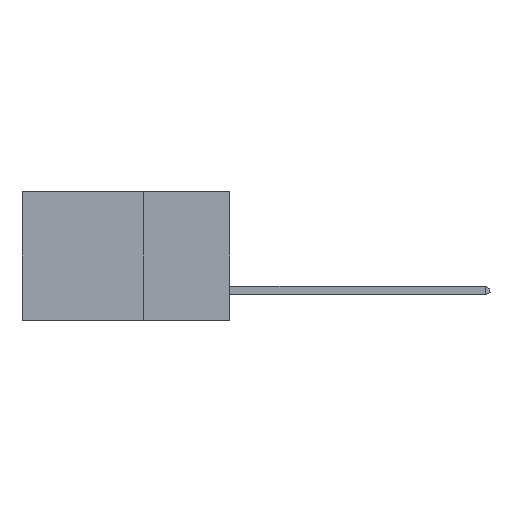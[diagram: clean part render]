
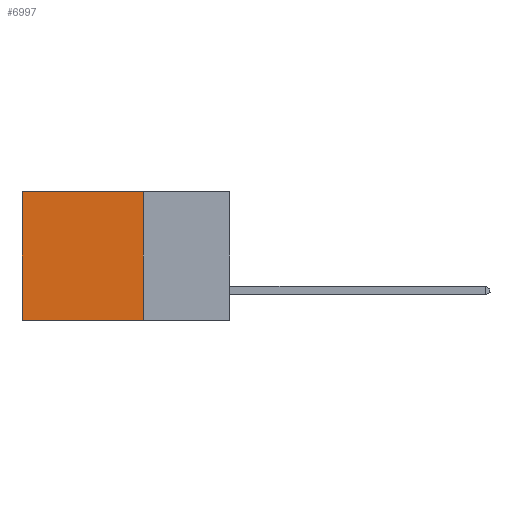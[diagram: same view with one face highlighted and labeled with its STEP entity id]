
A CAD part, left-side view. The second image highlights one B-rep face of the part: STEP entity #6997.
In plain terms, the highlighted planar face has unit normal (-1, 0, 0).
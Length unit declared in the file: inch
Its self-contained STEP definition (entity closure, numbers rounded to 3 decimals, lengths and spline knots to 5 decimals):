
#218 = VECTOR ( 'NONE', #5880, 39.37008 ) ;
#283 = VERTEX_POINT ( 'NONE', #2906 ) ;
#334 = ORIENTED_EDGE ( 'NONE', *, *, #6872, .T. ) ;
#347 = EDGE_LOOP ( 'NONE', ( #334, #7657, #8997, #8576 ) ) ;
#611 = DIRECTION ( 'NONE',  ( 0., 0., -1. ) ) ;
#1597 = PLANE ( 'NONE',  #7662 ) ;
#2161 = VECTOR ( 'NONE', #611, 39.37008 ) ;
#2418 = EDGE_CURVE ( 'NONE', #10155, #283, #3100, .T. ) ;
#2512 = LINE ( 'NONE', #2868, #4429 ) ;
#2868 = CARTESIAN_POINT ( 'NONE',  ( 0.298, 0.25, 0. ) ) ;
#2906 = CARTESIAN_POINT ( 'NONE',  ( 0.298, 0.6, -0.37 ) ) ;
#3100 = LINE ( 'NONE', #10220, #218 ) ;
#3622 = LINE ( 'NONE', #8442, #11335 ) ;
#4429 = VECTOR ( 'NONE', #8259, 39.37008 ) ;
#4506 = LINE ( 'NONE', #7563, #2161 ) ;
#5322 = CARTESIAN_POINT ( 'NONE',  ( 0.298, 0.25, -0.37 ) ) ;
#5880 = DIRECTION ( 'NONE',  ( 0., 1., 0. ) ) ;
#5941 = DIRECTION ( 'NONE',  ( 1., 0., 0. ) ) ;
#6252 = CARTESIAN_POINT ( 'NONE',  ( 0.298, 0.25, 0. ) ) ;
#6748 = DIRECTION ( 'NONE',  ( 0., 0., -1. ) ) ;
#6833 = DIRECTION ( 'NONE',  ( 0., 0., -1. ) ) ;
#6872 = EDGE_CURVE ( 'NONE', #8047, #283, #4506, .T. ) ;
#6997 = ADVANCED_FACE ( 'NONE', ( #10555 ), #1597, .F. ) ;
#7149 = CARTESIAN_POINT ( 'NONE',  ( 0.298, 0.6, 0. ) ) ;
#7563 = CARTESIAN_POINT ( 'NONE',  ( 0.298, 0.6, 0. ) ) ;
#7657 = ORIENTED_EDGE ( 'NONE', *, *, #2418, .F. ) ;
#7662 = AXIS2_PLACEMENT_3D ( 'NONE', #7779, #5941, #6833 ) ;
#7779 = CARTESIAN_POINT ( 'NONE',  ( 0.298, 0.25, 0. ) ) ;
#8047 = VERTEX_POINT ( 'NONE', #7149 ) ;
#8259 = DIRECTION ( 'NONE',  ( 0., 1., 0. ) ) ;
#8322 = VERTEX_POINT ( 'NONE', #6252 ) ;
#8442 = CARTESIAN_POINT ( 'NONE',  ( 0.298, 0.25, 0. ) ) ;
#8538 = EDGE_CURVE ( 'NONE', #8322, #10155, #3622, .T. ) ;
#8576 = ORIENTED_EDGE ( 'NONE', *, *, #10194, .T. ) ;
#8997 = ORIENTED_EDGE ( 'NONE', *, *, #8538, .F. ) ;
#10155 = VERTEX_POINT ( 'NONE', #5322 ) ;
#10194 = EDGE_CURVE ( 'NONE', #8322, #8047, #2512, .T. ) ;
#10220 = CARTESIAN_POINT ( 'NONE',  ( 0.298, 0.25, -0.37 ) ) ;
#10555 = FACE_OUTER_BOUND ( 'NONE', #347, .T. ) ;
#11335 = VECTOR ( 'NONE', #6748, 39.37008 ) ;
